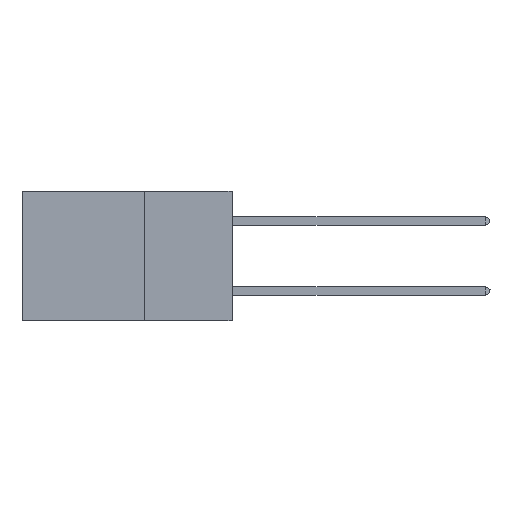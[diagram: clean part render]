
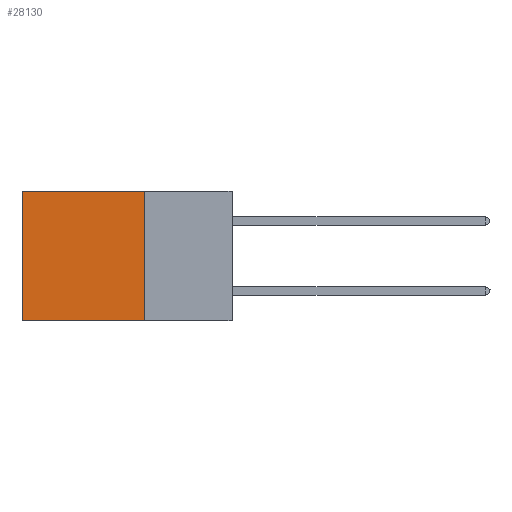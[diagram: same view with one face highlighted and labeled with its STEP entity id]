
A CAD part, left-side view. The second image highlights one B-rep face of the part: STEP entity #28130.
In plain terms, the highlighted planar face has unit normal (-1, 0, 0).
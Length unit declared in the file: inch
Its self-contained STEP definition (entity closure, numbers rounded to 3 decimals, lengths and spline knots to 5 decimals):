
#1408 = DIRECTION ( 'NONE',  ( 0., 0., -1. ) ) ;
#2383 = EDGE_CURVE ( 'NONE', #6248, #12635, #20480, .T. ) ;
#2691 = VERTEX_POINT ( 'NONE', #27020 ) ;
#2762 = DIRECTION ( 'NONE',  ( 0., 1., 0. ) ) ;
#3960 = PLANE ( 'NONE',  #26036 ) ;
#4261 = DIRECTION ( 'NONE',  ( 0., 0., -1. ) ) ;
#5823 = CARTESIAN_POINT ( 'NONE',  ( 0.2875, 0.6, 0. ) ) ;
#6248 = VERTEX_POINT ( 'NONE', #7052 ) ;
#7052 = CARTESIAN_POINT ( 'NONE',  ( 0.2875, 0.25, -0.37 ) ) ;
#7620 = VECTOR ( 'NONE', #11455, 39.37008 ) ;
#8610 = DIRECTION ( 'NONE',  ( 0., 0., -1. ) ) ;
#9628 = LINE ( 'NONE', #18490, #20098 ) ;
#11129 = CARTESIAN_POINT ( 'NONE',  ( 0.2875, 0.25, 0. ) ) ;
#11455 = DIRECTION ( 'NONE',  ( 0., 1., 0. ) ) ;
#12635 = VERTEX_POINT ( 'NONE', #15172 ) ;
#12786 = ORIENTED_EDGE ( 'NONE', *, *, #17503, .F. ) ;
#15172 = CARTESIAN_POINT ( 'NONE',  ( 0.2875, 0.6, -0.37 ) ) ;
#15328 = LINE ( 'NONE', #15786, #26153 ) ;
#15786 = CARTESIAN_POINT ( 'NONE',  ( 0.2875, 0.25, 0. ) ) ;
#16530 = EDGE_CURVE ( 'NONE', #2691, #12635, #20022, .T. ) ;
#17503 = EDGE_CURVE ( 'NONE', #22604, #6248, #15328, .T. ) ;
#17527 = ORIENTED_EDGE ( 'NONE', *, *, #2383, .F. ) ;
#18344 = EDGE_LOOP ( 'NONE', ( #27631, #17527, #12786, #28079 ) ) ;
#18490 = CARTESIAN_POINT ( 'NONE',  ( 0.2875, 0.25, 0. ) ) ;
#20022 = LINE ( 'NONE', #5823, #24710 ) ;
#20098 = VECTOR ( 'NONE', #2762, 39.37008 ) ;
#20442 = DIRECTION ( 'NONE',  ( 1., 0., 0. ) ) ;
#20480 = LINE ( 'NONE', #29951, #7620 ) ;
#22579 = FACE_OUTER_BOUND ( 'NONE', #18344, .T. ) ;
#22604 = VERTEX_POINT ( 'NONE', #24747 ) ;
#24710 = VECTOR ( 'NONE', #1408, 39.37008 ) ;
#24747 = CARTESIAN_POINT ( 'NONE',  ( 0.2875, 0.25, 0. ) ) ;
#26036 = AXIS2_PLACEMENT_3D ( 'NONE', #11129, #20442, #4261 ) ;
#26153 = VECTOR ( 'NONE', #8610, 39.37008 ) ;
#26604 = EDGE_CURVE ( 'NONE', #22604, #2691, #9628, .T. ) ;
#27020 = CARTESIAN_POINT ( 'NONE',  ( 0.2875, 0.6, 0. ) ) ;
#27631 = ORIENTED_EDGE ( 'NONE', *, *, #16530, .T. ) ;
#28079 = ORIENTED_EDGE ( 'NONE', *, *, #26604, .T. ) ;
#28130 = ADVANCED_FACE ( 'NONE', ( #22579 ), #3960, .F. ) ;
#29951 = CARTESIAN_POINT ( 'NONE',  ( 0.2875, 0.25, -0.37 ) ) ;
